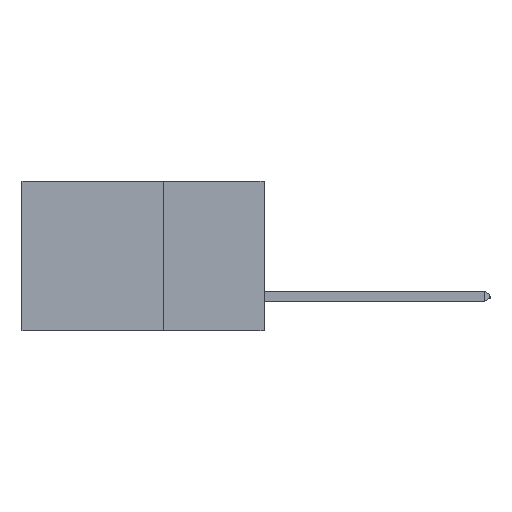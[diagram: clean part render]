
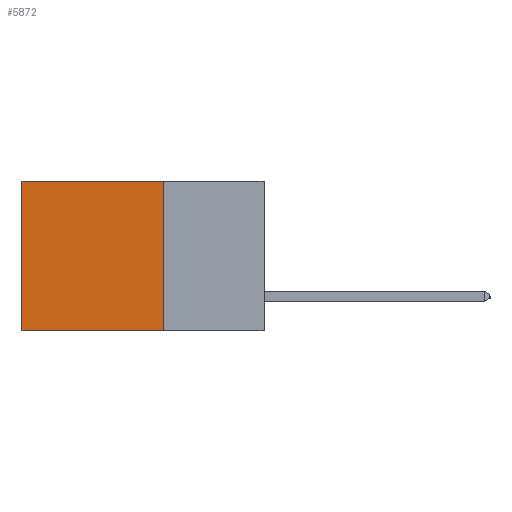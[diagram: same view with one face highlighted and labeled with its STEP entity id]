
A CAD part, left-side view. The second image highlights one B-rep face of the part: STEP entity #5872.
In plain terms, the highlighted planar face has unit normal (-1, 0, 0).
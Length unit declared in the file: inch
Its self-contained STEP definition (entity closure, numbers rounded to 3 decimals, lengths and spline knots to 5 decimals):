
#971 = EDGE_CURVE ( 'NONE', #10590, #8414, #23969, .T. ) ;
#1160 = EDGE_LOOP ( 'NONE', ( #14430, #6865, #10399, #20653 ) ) ;
#1307 = EDGE_CURVE ( 'NONE', #8414, #1692, #6126, .T. ) ;
#1667 = DIRECTION ( 'NONE',  ( 0., 0., -1. ) ) ;
#1692 = VERTEX_POINT ( 'NONE', #18894 ) ;
#3218 = DIRECTION ( 'NONE',  ( 0., 0., -1. ) ) ;
#5288 = CARTESIAN_POINT ( 'NONE',  ( 0.298, 0.25, -0.37 ) ) ;
#5872 = ADVANCED_FACE ( 'NONE', ( #14553 ), #6777, .F. ) ;
#6126 = LINE ( 'NONE', #11983, #20682 ) ;
#6285 = VECTOR ( 'NONE', #1667, 39.37008 ) ;
#6777 = PLANE ( 'NONE',  #24487 ) ;
#6865 = ORIENTED_EDGE ( 'NONE', *, *, #11999, .F. ) ;
#6900 = LINE ( 'NONE', #25349, #6285 ) ;
#7780 = CARTESIAN_POINT ( 'NONE',  ( 0.298, 0.25, -0.37 ) ) ;
#8414 = VERTEX_POINT ( 'NONE', #24608 ) ;
#8708 = EDGE_CURVE ( 'NONE', #10590, #11837, #6900, .T. ) ;
#8792 = DIRECTION ( 'NONE',  ( 1., 0., 0. ) ) ;
#10013 = CARTESIAN_POINT ( 'NONE',  ( 0.298, 0.25, 0. ) ) ;
#10399 = ORIENTED_EDGE ( 'NONE', *, *, #8708, .F. ) ;
#10483 = DIRECTION ( 'NONE',  ( 0., 1., 0. ) ) ;
#10590 = VERTEX_POINT ( 'NONE', #20352 ) ;
#11837 = VERTEX_POINT ( 'NONE', #5288 ) ;
#11983 = CARTESIAN_POINT ( 'NONE',  ( 0.298, 0.6, 0. ) ) ;
#11999 = EDGE_CURVE ( 'NONE', #11837, #1692, #21040, .T. ) ;
#13000 = VECTOR ( 'NONE', #10483, 39.37008 ) ;
#14430 = ORIENTED_EDGE ( 'NONE', *, *, #1307, .T. ) ;
#14553 = FACE_OUTER_BOUND ( 'NONE', #1160, .T. ) ;
#16445 = VECTOR ( 'NONE', #21593, 39.37008 ) ;
#18728 = CARTESIAN_POINT ( 'NONE',  ( 0.298, 0.25, 0. ) ) ;
#18894 = CARTESIAN_POINT ( 'NONE',  ( 0.298, 0.6, -0.37 ) ) ;
#20352 = CARTESIAN_POINT ( 'NONE',  ( 0.298, 0.25, 0. ) ) ;
#20653 = ORIENTED_EDGE ( 'NONE', *, *, #971, .T. ) ;
#20682 = VECTOR ( 'NONE', #3218, 39.37008 ) ;
#21040 = LINE ( 'NONE', #7780, #16445 ) ;
#21593 = DIRECTION ( 'NONE',  ( 0., 1., 0. ) ) ;
#22564 = DIRECTION ( 'NONE',  ( 0., 0., -1. ) ) ;
#23969 = LINE ( 'NONE', #10013, #13000 ) ;
#24487 = AXIS2_PLACEMENT_3D ( 'NONE', #18728, #8792, #22564 ) ;
#24608 = CARTESIAN_POINT ( 'NONE',  ( 0.298, 0.6, 0. ) ) ;
#25349 = CARTESIAN_POINT ( 'NONE',  ( 0.298, 0.25, 0. ) ) ;
